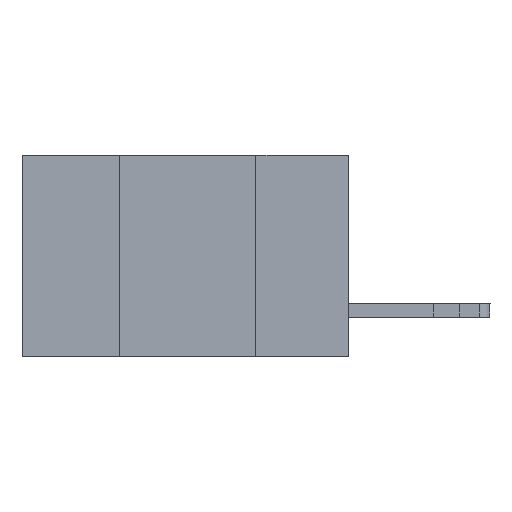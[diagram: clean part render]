
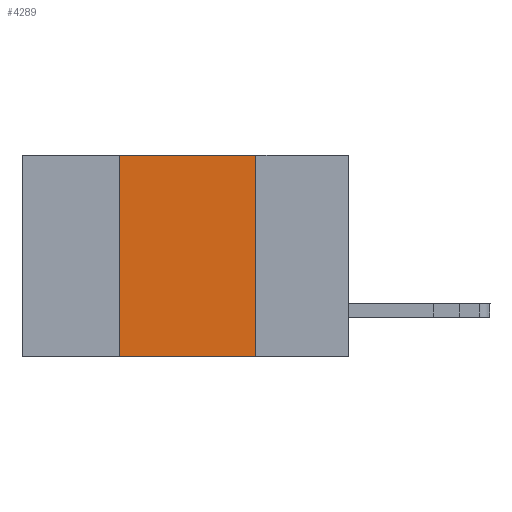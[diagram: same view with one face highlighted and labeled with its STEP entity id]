
A CAD part, left-side view. The second image highlights one B-rep face of the part: STEP entity #4289.
In plain terms, the highlighted planar face has unit normal (-1, 0, 0).
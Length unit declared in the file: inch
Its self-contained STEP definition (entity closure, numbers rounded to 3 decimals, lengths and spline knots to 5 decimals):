
#91 = FACE_OUTER_BOUND ( 'NONE', #6818, .T. ) ;
#470 = EDGE_CURVE ( 'NONE', #12052, #1112, #1339, .T. ) ;
#1041 = CARTESIAN_POINT ( 'NONE',  ( 0., 0.17, 0. ) ) ;
#1112 = VERTEX_POINT ( 'NONE', #3916 ) ;
#1339 = LINE ( 'NONE', #9555, #15216 ) ;
#2674 = LINE ( 'NONE', #1041, #7477 ) ;
#2794 = CARTESIAN_POINT ( 'NONE',  ( 0., 0.6, -0.37 ) ) ;
#2992 = DIRECTION ( 'NONE',  ( 0., 0., 1. ) ) ;
#3462 = DIRECTION ( 'NONE',  ( 0., 0., -1. ) ) ;
#3916 = CARTESIAN_POINT ( 'NONE',  ( 0., 0.17, 0. ) ) ;
#4273 = VERTEX_POINT ( 'NONE', #11937 ) ;
#4289 = ADVANCED_FACE ( 'NONE', ( #91 ), #8375, .F. ) ;
#4799 = DIRECTION ( 'NONE',  ( 1., 0., 0. ) ) ;
#5636 = VERTEX_POINT ( 'NONE', #14367 ) ;
#6707 = ORIENTED_EDGE ( 'NONE', *, *, #470, .F. ) ;
#6818 = EDGE_LOOP ( 'NONE', ( #14230, #6707, #12014, #9403 ) ) ;
#7042 = VECTOR ( 'NONE', #2992, 39.37008 ) ;
#7279 = DIRECTION ( 'NONE',  ( 0., 0., -1. ) ) ;
#7477 = VECTOR ( 'NONE', #3462, 39.37008 ) ;
#7775 = LINE ( 'NONE', #2794, #13373 ) ;
#7849 = CARTESIAN_POINT ( 'NONE',  ( 0., 0.42, 0. ) ) ;
#8030 = EDGE_CURVE ( 'NONE', #4273, #5636, #7775, .T. ) ;
#8065 = EDGE_CURVE ( 'NONE', #4273, #12052, #12105, .T. ) ;
#8375 = PLANE ( 'NONE',  #11116 ) ;
#9403 = ORIENTED_EDGE ( 'NONE', *, *, #8030, .T. ) ;
#9555 = CARTESIAN_POINT ( 'NONE',  ( 0., 0.6, 0. ) ) ;
#9795 = DIRECTION ( 'NONE',  ( 0., -1., 0. ) ) ;
#10782 = DIRECTION ( 'NONE',  ( 0., -1., 0. ) ) ;
#11116 = AXIS2_PLACEMENT_3D ( 'NONE', #14395, #4799, #7279 ) ;
#11937 = CARTESIAN_POINT ( 'NONE',  ( 0., 0.42, -0.37 ) ) ;
#12014 = ORIENTED_EDGE ( 'NONE', *, *, #8065, .F. ) ;
#12052 = VERTEX_POINT ( 'NONE', #12711 ) ;
#12105 = LINE ( 'NONE', #7849, #7042 ) ;
#12548 = EDGE_CURVE ( 'NONE', #1112, #5636, #2674, .T. ) ;
#12711 = CARTESIAN_POINT ( 'NONE',  ( 0., 0.42, 0. ) ) ;
#13373 = VECTOR ( 'NONE', #9795, 39.37008 ) ;
#14230 = ORIENTED_EDGE ( 'NONE', *, *, #12548, .F. ) ;
#14367 = CARTESIAN_POINT ( 'NONE',  ( 0., 0.17, -0.37 ) ) ;
#14395 = CARTESIAN_POINT ( 'NONE',  ( 0., 0.6, 0. ) ) ;
#15216 = VECTOR ( 'NONE', #10782, 39.37008 ) ;
